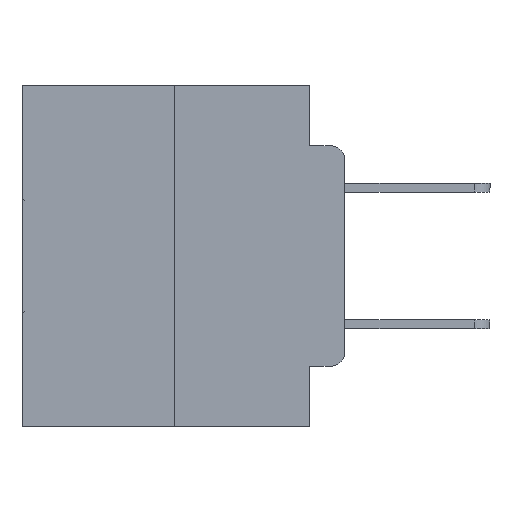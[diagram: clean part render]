
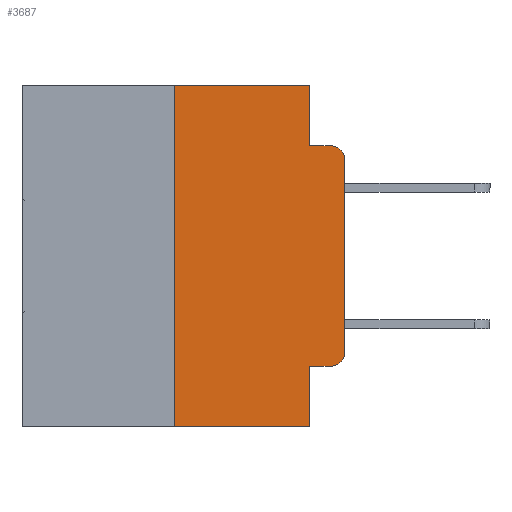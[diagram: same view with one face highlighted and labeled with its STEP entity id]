
A CAD part, left-side view. The second image highlights one B-rep face of the part: STEP entity #3687.
In plain terms, the highlighted planar face has unit normal (-1, 0, 0).
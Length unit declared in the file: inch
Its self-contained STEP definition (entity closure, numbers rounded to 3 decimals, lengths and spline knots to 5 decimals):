
#162 = EDGE_CURVE ( 'NONE', #27477, #23420, #19090, .T. ) ;
#446 = CARTESIAN_POINT ( 'NONE',  ( 0., 0.02, -0.4115 ) ) ;
#1040 = ORIENTED_EDGE ( 'NONE', *, *, #22833, .F. ) ;
#1107 = LINE ( 'NONE', #12669, #8043 ) ;
#1173 = AXIS2_PLACEMENT_3D ( 'NONE', #13984, #30419, #16377 ) ;
#1501 = CARTESIAN_POINT ( 'NONE',  ( 0., 0.051, 0. ) ) ;
#1517 = LINE ( 'NONE', #9592, #6271 ) ;
#1718 = AXIS2_PLACEMENT_3D ( 'NONE', #12413, #28870, #14778 ) ;
#1738 = EDGE_CURVE ( 'NONE', #23420, #15782, #8535, .T. ) ;
#1790 = VERTEX_POINT ( 'NONE', #20854 ) ;
#2748 = CARTESIAN_POINT ( 'NONE',  ( 0., 0.051, 0. ) ) ;
#2842 = CARTESIAN_POINT ( 'NONE',  ( 0., 0.02, -0.0885 ) ) ;
#2890 = ORIENTED_EDGE ( 'NONE', *, *, #3766, .T. ) ;
#3401 = EDGE_CURVE ( 'NONE', #30282, #27477, #1107, .T. ) ;
#3630 = ORIENTED_EDGE ( 'NONE', *, *, #1738, .F. ) ;
#3687 = ADVANCED_FACE ( 'NONE', ( #17263 ), #4287, .F. ) ;
#3766 = EDGE_CURVE ( 'NONE', #1790, #15782, #15033, .T. ) ;
#4287 = PLANE ( 'NONE',  #30092 ) ;
#5097 = ORIENTED_EDGE ( 'NONE', *, *, #24397, .F. ) ;
#5653 = VECTOR ( 'NONE', #21415, 39.37008 ) ;
#5686 = CARTESIAN_POINT ( 'NONE',  ( 0., 0.25, 0. ) ) ;
#6131 = DIRECTION ( 'NONE',  ( 0., 0., 1. ) ) ;
#6236 = VERTEX_POINT ( 'NONE', #9629 ) ;
#6271 = VECTOR ( 'NONE', #19058, 39.37008 ) ;
#6478 = VECTOR ( 'NONE', #6131, 39.37008 ) ;
#6518 = ORIENTED_EDGE ( 'NONE', *, *, #11996, .T. ) ;
#8043 = VECTOR ( 'NONE', #17332, 39.37008 ) ;
#8138 = CARTESIAN_POINT ( 'NONE',  ( 0., 0.25, 0. ) ) ;
#8177 = EDGE_LOOP ( 'NONE', ( #20160, #2890, #3630, #9845, #16111, #5097, #6518, #1040, #26778, #9474 ) ) ;
#8435 = EDGE_CURVE ( 'NONE', #19151, #1790, #12009, .T. ) ;
#8535 = LINE ( 'NONE', #23948, #21817 ) ;
#9474 = ORIENTED_EDGE ( 'NONE', *, *, #16515, .T. ) ;
#9592 = CARTESIAN_POINT ( 'NONE',  ( 0., 0.473, -0.5 ) ) ;
#9629 = CARTESIAN_POINT ( 'NONE',  ( 0., 0.25, -0.5 ) ) ;
#9845 = ORIENTED_EDGE ( 'NONE', *, *, #162, .F. ) ;
#10894 = CIRCLE ( 'NONE', #1718, 0.02 ) ;
#11393 = LINE ( 'NONE', #8138, #12146 ) ;
#11996 = EDGE_CURVE ( 'NONE', #6236, #26231, #1517, .T. ) ;
#12009 = LINE ( 'NONE', #22702, #6478 ) ;
#12146 = VECTOR ( 'NONE', #22267, 39.37008 ) ;
#12413 = CARTESIAN_POINT ( 'NONE',  ( 0., 0.02, -0.3915 ) ) ;
#12669 = CARTESIAN_POINT ( 'NONE',  ( 0., 0.473, 0. ) ) ;
#12811 = VECTOR ( 'NONE', #24168, 39.37008 ) ;
#12827 = DIRECTION ( 'NONE',  ( 0., -1., 0. ) ) ;
#13674 = DIRECTION ( 'NONE',  ( 1., 0., 0. ) ) ;
#13984 = CARTESIAN_POINT ( 'NONE',  ( 0., 0.02, -0.1085 ) ) ;
#14778 = DIRECTION ( 'NONE',  ( 0., 0., -1. ) ) ;
#15033 = CIRCLE ( 'NONE', #1173, 0.02 ) ;
#15628 = VERTEX_POINT ( 'NONE', #23393 ) ;
#15782 = VERTEX_POINT ( 'NONE', #2842 ) ;
#16111 = ORIENTED_EDGE ( 'NONE', *, *, #3401, .F. ) ;
#16186 = DIRECTION ( 'NONE',  ( 0., -1., 0. ) ) ;
#16377 = DIRECTION ( 'NONE',  ( 0., 0., -1. ) ) ;
#16515 = EDGE_CURVE ( 'NONE', #22872, #19151, #10894, .T. ) ;
#17263 = FACE_OUTER_BOUND ( 'NONE', #8177, .T. ) ;
#17332 = DIRECTION ( 'NONE',  ( 0., -1., 0. ) ) ;
#17401 = LINE ( 'NONE', #28484, #5653 ) ;
#18584 = VECTOR ( 'NONE', #12827, 39.37008 ) ;
#18888 = CARTESIAN_POINT ( 'NONE',  ( 0., 0.051, -0.0885 ) ) ;
#19058 = DIRECTION ( 'NONE',  ( 0., -1., 0. ) ) ;
#19090 = LINE ( 'NONE', #1501, #12811 ) ;
#19151 = VERTEX_POINT ( 'NONE', #26281 ) ;
#20011 = CARTESIAN_POINT ( 'NONE',  ( 0., 0.051, -0.5 ) ) ;
#20104 = LINE ( 'NONE', #22226, #18584 ) ;
#20160 = ORIENTED_EDGE ( 'NONE', *, *, #8435, .T. ) ;
#20854 = CARTESIAN_POINT ( 'NONE',  ( 0., 0., -0.1085 ) ) ;
#21239 = EDGE_CURVE ( 'NONE', #15628, #22872, #20104, .T. ) ;
#21415 = DIRECTION ( 'NONE',  ( 0., 0., -1. ) ) ;
#21817 = VECTOR ( 'NONE', #16186, 39.37008 ) ;
#22226 = CARTESIAN_POINT ( 'NONE',  ( 0., 0.051, -0.4115 ) ) ;
#22267 = DIRECTION ( 'NONE',  ( 0., 0., 1. ) ) ;
#22702 = CARTESIAN_POINT ( 'NONE',  ( 0., 0., 0. ) ) ;
#22833 = EDGE_CURVE ( 'NONE', #15628, #26231, #17401, .T. ) ;
#22872 = VERTEX_POINT ( 'NONE', #446 ) ;
#23080 = CARTESIAN_POINT ( 'NONE',  ( 0., 0.473, 0. ) ) ;
#23393 = CARTESIAN_POINT ( 'NONE',  ( 0., 0.051, -0.4115 ) ) ;
#23420 = VERTEX_POINT ( 'NONE', #18888 ) ;
#23948 = CARTESIAN_POINT ( 'NONE',  ( 0., 0.051, -0.0885 ) ) ;
#24168 = DIRECTION ( 'NONE',  ( 0., 0., -1. ) ) ;
#24397 = EDGE_CURVE ( 'NONE', #6236, #30282, #11393, .T. ) ;
#26231 = VERTEX_POINT ( 'NONE', #20011 ) ;
#26281 = CARTESIAN_POINT ( 'NONE',  ( 0., 0., -0.3915 ) ) ;
#26778 = ORIENTED_EDGE ( 'NONE', *, *, #21239, .T. ) ;
#27477 = VERTEX_POINT ( 'NONE', #2748 ) ;
#28484 = CARTESIAN_POINT ( 'NONE',  ( 0., 0.051, 0. ) ) ;
#28870 = DIRECTION ( 'NONE',  ( -1., 0., 0. ) ) ;
#30092 = AXIS2_PLACEMENT_3D ( 'NONE', #23080, #13674, #30130 ) ;
#30130 = DIRECTION ( 'NONE',  ( 0., 0., -1. ) ) ;
#30282 = VERTEX_POINT ( 'NONE', #5686 ) ;
#30419 = DIRECTION ( 'NONE',  ( -1., 0., 0. ) ) ;
